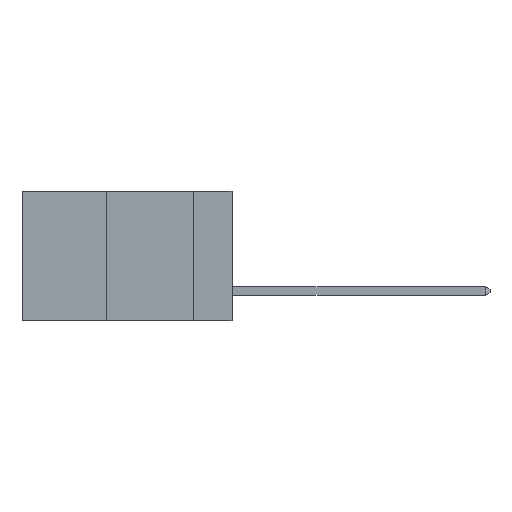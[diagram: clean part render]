
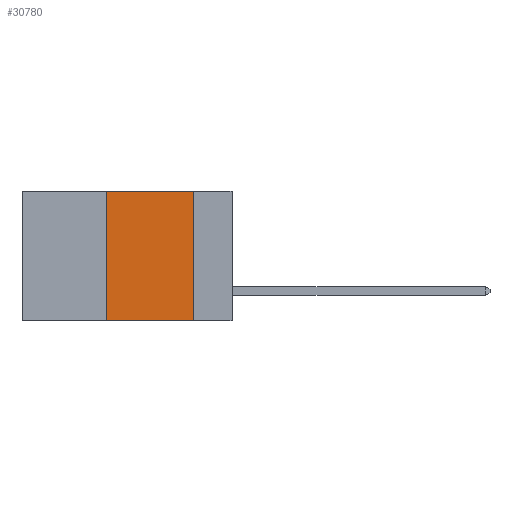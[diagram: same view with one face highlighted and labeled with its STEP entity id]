
A CAD part, left-side view. The second image highlights one B-rep face of the part: STEP entity #30780.
In plain terms, the highlighted planar face has unit normal (-1, 0, 0).
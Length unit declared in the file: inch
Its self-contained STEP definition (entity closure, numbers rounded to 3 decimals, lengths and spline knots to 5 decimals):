
#80 = EDGE_CURVE ( 'NONE', #7926, #3128, #317, .T. ) ;
#317 = LINE ( 'NONE', #29994, #18743 ) ;
#395 = DIRECTION ( 'NONE',  ( 0., 0., -1. ) ) ;
#1938 = VECTOR ( 'NONE', #21076, 39.37008 ) ;
#2765 = LINE ( 'NONE', #10680, #1938 ) ;
#3128 = VERTEX_POINT ( 'NONE', #28050 ) ;
#3262 = CARTESIAN_POINT ( 'NONE',  ( 0., 0.36, -0.37 ) ) ;
#7220 = CARTESIAN_POINT ( 'NONE',  ( 0., 0.36, 0. ) ) ;
#7926 = VERTEX_POINT ( 'NONE', #3262 ) ;
#8044 = VECTOR ( 'NONE', #12605, 39.37008 ) ;
#9814 = EDGE_CURVE ( 'NONE', #32537, #3128, #19827, .T. ) ;
#10680 = CARTESIAN_POINT ( 'NONE',  ( 0., 0.6, 0. ) ) ;
#12605 = DIRECTION ( 'NONE',  ( 0., 0., 1. ) ) ;
#12937 = FACE_OUTER_BOUND ( 'NONE', #16455, .T. ) ;
#13980 = EDGE_CURVE ( 'NONE', #32013, #32537, #2765, .T. ) ;
#14941 = LINE ( 'NONE', #30676, #8044 ) ;
#14969 = CARTESIAN_POINT ( 'NONE',  ( 0., 0.6, 0. ) ) ;
#16455 = EDGE_LOOP ( 'NONE', ( #23758, #18180, #26546, #29927 ) ) ;
#17573 = DIRECTION ( 'NONE',  ( 0., 0., -1. ) ) ;
#18123 = EDGE_CURVE ( 'NONE', #7926, #32013, #14941, .T. ) ;
#18180 = ORIENTED_EDGE ( 'NONE', *, *, #13980, .F. ) ;
#18743 = VECTOR ( 'NONE', #30057, 39.37008 ) ;
#19827 = LINE ( 'NONE', #31523, #25094 ) ;
#21076 = DIRECTION ( 'NONE',  ( 0., -1., 0. ) ) ;
#21260 = AXIS2_PLACEMENT_3D ( 'NONE', #14969, #32944, #17573 ) ;
#23758 = ORIENTED_EDGE ( 'NONE', *, *, #9814, .F. ) ;
#24996 = CARTESIAN_POINT ( 'NONE',  ( 0., 0.11, 0. ) ) ;
#25094 = VECTOR ( 'NONE', #395, 39.37008 ) ;
#26546 = ORIENTED_EDGE ( 'NONE', *, *, #18123, .F. ) ;
#28050 = CARTESIAN_POINT ( 'NONE',  ( 0., 0.11, -0.37 ) ) ;
#29927 = ORIENTED_EDGE ( 'NONE', *, *, #80, .T. ) ;
#29994 = CARTESIAN_POINT ( 'NONE',  ( 0., 0.6, -0.37 ) ) ;
#30057 = DIRECTION ( 'NONE',  ( 0., -1., 0. ) ) ;
#30428 = PLANE ( 'NONE',  #21260 ) ;
#30676 = CARTESIAN_POINT ( 'NONE',  ( 0., 0.36, 0. ) ) ;
#30780 = ADVANCED_FACE ( 'NONE', ( #12937 ), #30428, .F. ) ;
#31523 = CARTESIAN_POINT ( 'NONE',  ( 0., 0.11, 0. ) ) ;
#32013 = VERTEX_POINT ( 'NONE', #7220 ) ;
#32537 = VERTEX_POINT ( 'NONE', #24996 ) ;
#32944 = DIRECTION ( 'NONE',  ( 1., 0., 0. ) ) ;
